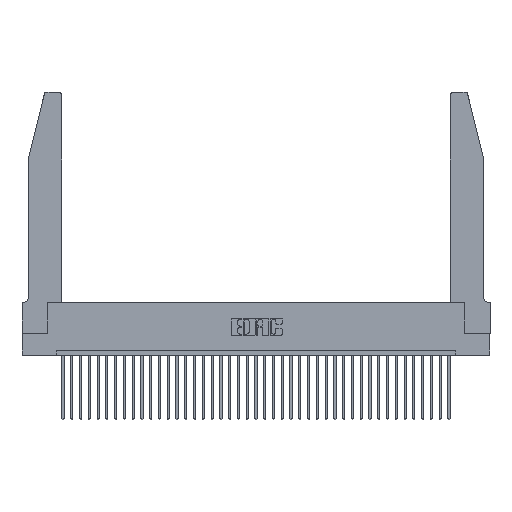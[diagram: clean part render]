
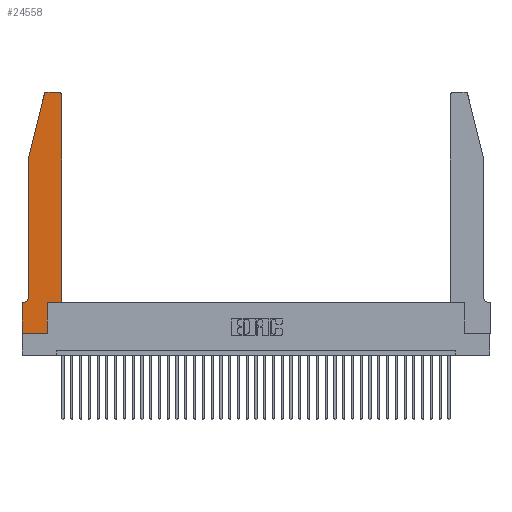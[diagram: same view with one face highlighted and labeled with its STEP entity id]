
A CAD part, top view. The second image highlights one B-rep face of the part: STEP entity #24558.
In plain terms, the highlighted planar face has unit normal (0, 0, 1).
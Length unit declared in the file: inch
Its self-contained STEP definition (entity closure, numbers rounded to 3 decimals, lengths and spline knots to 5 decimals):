
#959 = VERTEX_POINT ( 'NONE', #6381 ) ;
#1737 = VERTEX_POINT ( 'NONE', #24507 ) ;
#1740 = CARTESIAN_POINT ( 'NONE',  ( 0.4505, 0.35, 0.37 ) ) ;
#2601 = VECTOR ( 'NONE', #19637, 39.37008 ) ;
#3272 = VERTEX_POINT ( 'NONE', #1740 ) ;
#3711 = LINE ( 'NONE', #14810, #19354 ) ;
#3796 = CARTESIAN_POINT ( 'NONE',  ( 0.0055, 0.35, 0.37 ) ) ;
#3967 = VERTEX_POINT ( 'NONE', #24246 ) ;
#4316 = DIRECTION ( 'NONE',  ( 1., 0., 0. ) ) ;
#4430 = DIRECTION ( 'NONE',  ( 0., 0., -1. ) ) ;
#4801 = VERTEX_POINT ( 'NONE', #3796 ) ;
#5474 = DIRECTION ( 'NONE',  ( 0., 1., 0. ) ) ;
#5763 = VECTOR ( 'NONE', #31437, 39.37008 ) ;
#5926 = ORIENTED_EDGE ( 'NONE', *, *, #23714, .T. ) ;
#6381 = CARTESIAN_POINT ( 'NONE',  ( 0.2865, 0., 0.37 ) ) ;
#6560 = ORIENTED_EDGE ( 'NONE', *, *, #15823, .T. ) ;
#6667 = LINE ( 'NONE', #7754, #5763 ) ;
#6789 = CIRCLE ( 'NONE', #9757, 0.03 ) ;
#7413 = ORIENTED_EDGE ( 'NONE', *, *, #22075, .T. ) ;
#7499 = VECTOR ( 'NONE', #4316, 39.37008 ) ;
#7683 = CARTESIAN_POINT ( 'NONE',  ( 0.4505, 0.35, 0.37 ) ) ;
#7754 = CARTESIAN_POINT ( 'NONE',  ( 0.0755, 2., 0.37 ) ) ;
#7985 = AXIS2_PLACEMENT_3D ( 'NONE', #37249, #37633, #13821 ) ;
#9258 = EDGE_CURVE ( 'NONE', #3272, #12390, #34573, .T. ) ;
#9662 = VERTEX_POINT ( 'NONE', #24689 ) ;
#9688 = CARTESIAN_POINT ( 'NONE',  ( 0.0755, 2., 0.37 ) ) ;
#9757 = AXIS2_PLACEMENT_3D ( 'NONE', #26794, #29752, #15252 ) ;
#9937 = CARTESIAN_POINT ( 'NONE',  ( 0.0055, 0.42, 0.37 ) ) ;
#10860 = ORIENTED_EDGE ( 'NONE', *, *, #18611, .T. ) ;
#11501 = ORIENTED_EDGE ( 'NONE', *, *, #34538, .T. ) ;
#11635 = EDGE_CURVE ( 'NONE', #27823, #1737, #27089, .T. ) ;
#12203 = VERTEX_POINT ( 'NONE', #29626 ) ;
#12390 = VERTEX_POINT ( 'NONE', #35465 ) ;
#12987 = CARTESIAN_POINT ( 'NONE',  ( 0.2865, 0.35, 0.37 ) ) ;
#12991 = ORIENTED_EDGE ( 'NONE', *, *, #26702, .T. ) ;
#13531 = DIRECTION ( 'NONE',  ( 0., -1., 0. ) ) ;
#13821 = DIRECTION ( 'NONE',  ( 1., 0., 0. ) ) ;
#14324 = EDGE_CURVE ( 'NONE', #12203, #4801, #34240, .T. ) ;
#14810 = CARTESIAN_POINT ( 'NONE',  ( 0.0755, 0.35, 0.37 ) ) ;
#15252 = DIRECTION ( 'NONE',  ( 1., 0., 0. ) ) ;
#15823 = EDGE_CURVE ( 'NONE', #12390, #35735, #6789, .T. ) ;
#16017 = VECTOR ( 'NONE', #37653, 39.37008 ) ;
#16317 = PLANE ( 'NONE',  #7985 ) ;
#17412 = AXIS2_PLACEMENT_3D ( 'NONE', #9937, #4430, #22103 ) ;
#17419 = DIRECTION ( 'NONE',  ( -1., 0., 0. ) ) ;
#17667 = ORIENTED_EDGE ( 'NONE', *, *, #11635, .T. ) ;
#17746 = ORIENTED_EDGE ( 'NONE', *, *, #14324, .T. ) ;
#18006 = VECTOR ( 'NONE', #27746, 39.37008 ) ;
#18589 = ORIENTED_EDGE ( 'NONE', *, *, #30507, .T. ) ;
#18611 = EDGE_CURVE ( 'NONE', #24549, #3272, #25736, .T. ) ;
#19354 = VECTOR ( 'NONE', #32683, 39.37008 ) ;
#19637 = DIRECTION ( 'NONE',  ( -0.239, -0.971, 0. ) ) ;
#19718 = CARTESIAN_POINT ( 'NONE',  ( 0., 0., 0.37 ) ) ;
#19892 = DIRECTION ( 'NONE',  ( 1., 0., 0. ) ) ;
#20242 = CARTESIAN_POINT ( 'NONE',  ( 0.2605, 2.75, 0.37 ) ) ;
#20905 = LINE ( 'NONE', #35183, #7499 ) ;
#21273 = ORIENTED_EDGE ( 'NONE', *, *, #32333, .T. ) ;
#21708 = LINE ( 'NONE', #22308, #18006 ) ;
#21788 = EDGE_CURVE ( 'NONE', #27506, #959, #20905, .T. ) ;
#21993 = LINE ( 'NONE', #37091, #27993 ) ;
#22075 = EDGE_CURVE ( 'NONE', #9662, #27823, #26913, .T. ) ;
#22103 = DIRECTION ( 'NONE',  ( -1., 0., 0. ) ) ;
#22308 = CARTESIAN_POINT ( 'NONE',  ( 0.2865, 0.35, 0.37 ) ) ;
#23714 = EDGE_CURVE ( 'NONE', #1737, #12203, #6667, .T. ) ;
#24246 = CARTESIAN_POINT ( 'NONE',  ( 0., 0.35, 0.37 ) ) ;
#24507 = CARTESIAN_POINT ( 'NONE',  ( 0.0755, 2., 0.37 ) ) ;
#24549 = VERTEX_POINT ( 'NONE', #12987 ) ;
#24558 = ADVANCED_FACE ( 'NONE', ( #31089 ), #16317, .T. ) ;
#24689 = CARTESIAN_POINT ( 'NONE',  ( 0.284, 2.75, 0.37 ) ) ;
#25736 = LINE ( 'NONE', #7683, #16017 ) ;
#25978 = CARTESIAN_POINT ( 'NONE',  ( 0.4505, 0.35, 0.37 ) ) ;
#26498 = AXIS2_PLACEMENT_3D ( 'NONE', #28707, #37598, #19892 ) ;
#26702 = EDGE_CURVE ( 'NONE', #959, #24549, #21708, .T. ) ;
#26794 = CARTESIAN_POINT ( 'NONE',  ( 0.4205, 2.72, 0.37 ) ) ;
#26913 = CIRCLE ( 'NONE', #26498, 0.03 ) ;
#27089 = LINE ( 'NONE', #9688, #2601 ) ;
#27202 = EDGE_LOOP ( 'NONE', ( #18589, #7413, #17667, #5926, #17746, #21273, #11501, #32517, #12991, #10860, #28540, #6560 ) ) ;
#27506 = VERTEX_POINT ( 'NONE', #19718 ) ;
#27746 = DIRECTION ( 'NONE',  ( 0., 1., 0. ) ) ;
#27823 = VERTEX_POINT ( 'NONE', #36292 ) ;
#27993 = VECTOR ( 'NONE', #13531, 39.37008 ) ;
#28284 = LINE ( 'NONE', #20242, #33350 ) ;
#28366 = CARTESIAN_POINT ( 'NONE',  ( 0.4205, 2.75, 0.37 ) ) ;
#28540 = ORIENTED_EDGE ( 'NONE', *, *, #9258, .T. ) ;
#28707 = CARTESIAN_POINT ( 'NONE',  ( 0.284, 2.72, 0.37 ) ) ;
#29626 = CARTESIAN_POINT ( 'NONE',  ( 0.0755, 0.42, 0.37 ) ) ;
#29752 = DIRECTION ( 'NONE',  ( 0., 0., 1. ) ) ;
#30507 = EDGE_CURVE ( 'NONE', #35735, #9662, #28284, .T. ) ;
#31089 = FACE_OUTER_BOUND ( 'NONE', #27202, .T. ) ;
#31437 = DIRECTION ( 'NONE',  ( 0., -1., 0. ) ) ;
#31804 = VECTOR ( 'NONE', #5474, 39.37008 ) ;
#32333 = EDGE_CURVE ( 'NONE', #4801, #3967, #3711, .T. ) ;
#32517 = ORIENTED_EDGE ( 'NONE', *, *, #21788, .T. ) ;
#32683 = DIRECTION ( 'NONE',  ( -1., 0., 0. ) ) ;
#33350 = VECTOR ( 'NONE', #17419, 39.37008 ) ;
#34240 = CIRCLE ( 'NONE', #17412, 0.07 ) ;
#34538 = EDGE_CURVE ( 'NONE', #3967, #27506, #21993, .T. ) ;
#34573 = LINE ( 'NONE', #25978, #31804 ) ;
#35183 = CARTESIAN_POINT ( 'NONE',  ( 0., 0., 0.37 ) ) ;
#35465 = CARTESIAN_POINT ( 'NONE',  ( 0.4505, 2.72, 0.37 ) ) ;
#35735 = VERTEX_POINT ( 'NONE', #28366 ) ;
#36292 = CARTESIAN_POINT ( 'NONE',  ( 0.25487, 2.72718, 0.37 ) ) ;
#37091 = CARTESIAN_POINT ( 'NONE',  ( 0., 0., 0.37 ) ) ;
#37249 = CARTESIAN_POINT ( 'NONE',  ( 0., 0.35, 0.37 ) ) ;
#37598 = DIRECTION ( 'NONE',  ( 0., 0., 1. ) ) ;
#37633 = DIRECTION ( 'NONE',  ( 0., 0., 1. ) ) ;
#37653 = DIRECTION ( 'NONE',  ( 1., 0., 0. ) ) ;
